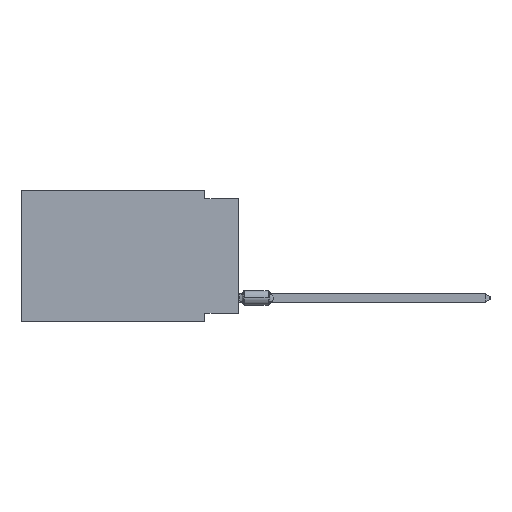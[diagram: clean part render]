
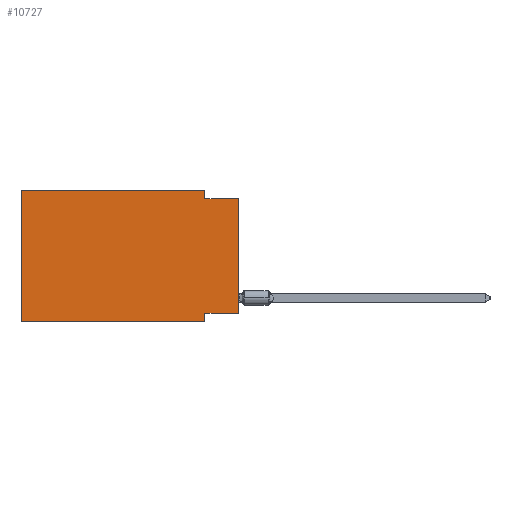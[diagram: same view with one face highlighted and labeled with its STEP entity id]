
A CAD part, left-side view. The second image highlights one B-rep face of the part: STEP entity #10727.
In plain terms, the highlighted planar face has unit normal (-1, 0, 0).
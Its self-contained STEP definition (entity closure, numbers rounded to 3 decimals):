
#38 = DIRECTION ( 'NONE',  ( 0., -1., 0. ) ) ;
#2158 = CARTESIAN_POINT ( 'NONE',  ( 0., 16.383, -9.906 ) ) ;
#3674 = LINE ( 'NONE', #37929, #44099 ) ;
#4008 = VECTOR ( 'NONE', #38, 1000. ) ;
#4027 = LINE ( 'NONE', #27089, #20086 ) ;
#5139 = CARTESIAN_POINT ( 'NONE',  ( 0., 0., -9.271 ) ) ;
#8320 = DIRECTION ( 'NONE',  ( 0., 0., 1. ) ) ;
#8462 = ORIENTED_EDGE ( 'NONE', *, *, #36257, .F. ) ;
#8533 = CARTESIAN_POINT ( 'NONE',  ( 0., 0., 0. ) ) ;
#8630 = DIRECTION ( 'NONE',  ( 1., 0., 0. ) ) ;
#8861 = FACE_OUTER_BOUND ( 'NONE', #24587, .T. ) ;
#9217 = ORIENTED_EDGE ( 'NONE', *, *, #28638, .F. ) ;
#10031 = VERTEX_POINT ( 'NONE', #24431 ) ;
#10727 = ADVANCED_FACE ( 'NONE', ( #8861 ), #39320, .F. ) ;
#11769 = CARTESIAN_POINT ( 'NONE',  ( 0., 16.383, 0. ) ) ;
#12430 = DIRECTION ( 'NONE',  ( 0., 0., -1. ) ) ;
#13097 = VECTOR ( 'NONE', #19785, 1000. ) ;
#13254 = VECTOR ( 'NONE', #38815, 1000. ) ;
#13742 = VECTOR ( 'NONE', #42339, 1000. ) ;
#15193 = ORIENTED_EDGE ( 'NONE', *, *, #21172, .F. ) ;
#15468 = EDGE_CURVE ( 'NONE', #16598, #10031, #3674, .T. ) ;
#16526 = ORIENTED_EDGE ( 'NONE', *, *, #15468, .F. ) ;
#16598 = VERTEX_POINT ( 'NONE', #39671 ) ;
#17488 = ORIENTED_EDGE ( 'NONE', *, *, #25750, .F. ) ;
#18610 = LINE ( 'NONE', #8533, #39622 ) ;
#18647 = CARTESIAN_POINT ( 'NONE',  ( 0., 16.383, 0. ) ) ;
#19785 = DIRECTION ( 'NONE',  ( 0., 1., 0. ) ) ;
#19995 = VERTEX_POINT ( 'NONE', #28957 ) ;
#20086 = VECTOR ( 'NONE', #20595, 1000. ) ;
#20595 = DIRECTION ( 'NONE',  ( 0., 0., -1. ) ) ;
#21172 = EDGE_CURVE ( 'NONE', #19995, #27235, #35238, .T. ) ;
#21295 = CARTESIAN_POINT ( 'NONE',  ( 0., 2.54, -9.906 ) ) ;
#21722 = CARTESIAN_POINT ( 'NONE',  ( 0., 2.54, -9.906 ) ) ;
#22419 = CARTESIAN_POINT ( 'NONE',  ( 0., 2.54, -9.271 ) ) ;
#23182 = CARTESIAN_POINT ( 'NONE',  ( 0., 16.383, 0. ) ) ;
#24431 = CARTESIAN_POINT ( 'NONE',  ( 0., 0., -0.635 ) ) ;
#24587 = EDGE_LOOP ( 'NONE', ( #43468, #16526, #17488, #9217, #15193, #35005, #26236, #8462 ) ) ;
#25228 = VERTEX_POINT ( 'NONE', #22419 ) ;
#25750 = EDGE_CURVE ( 'NONE', #42196, #16598, #4027, .T. ) ;
#26236 = ORIENTED_EDGE ( 'NONE', *, *, #33657, .F. ) ;
#27089 = CARTESIAN_POINT ( 'NONE',  ( 0., 2.54, 0. ) ) ;
#27235 = VERTEX_POINT ( 'NONE', #23182 ) ;
#28638 = EDGE_CURVE ( 'NONE', #27235, #42196, #36599, .T. ) ;
#28947 = VERTEX_POINT ( 'NONE', #5139 ) ;
#28957 = CARTESIAN_POINT ( 'NONE',  ( 0., 16.383, -9.906 ) ) ;
#29424 = VERTEX_POINT ( 'NONE', #21295 ) ;
#30718 = CARTESIAN_POINT ( 'NONE',  ( 0., 16.383, 0. ) ) ;
#31431 = DIRECTION ( 'NONE',  ( 0., -1., 0. ) ) ;
#31821 = EDGE_CURVE ( 'NONE', #19995, #29424, #35541, .T. ) ;
#32015 = AXIS2_PLACEMENT_3D ( 'NONE', #11769, #8630, #12430 ) ;
#33657 = EDGE_CURVE ( 'NONE', #25228, #29424, #42570, .T. ) ;
#33667 = CARTESIAN_POINT ( 'NONE',  ( 0., 0., -9.271 ) ) ;
#35005 = ORIENTED_EDGE ( 'NONE', *, *, #31821, .T. ) ;
#35238 = LINE ( 'NONE', #18647, #13254 ) ;
#35541 = LINE ( 'NONE', #2158, #40813 ) ;
#36257 = EDGE_CURVE ( 'NONE', #28947, #25228, #40408, .T. ) ;
#36599 = LINE ( 'NONE', #30718, #4008 ) ;
#37929 = CARTESIAN_POINT ( 'NONE',  ( 0., 0., -0.635 ) ) ;
#38815 = DIRECTION ( 'NONE',  ( 0., 0., 1. ) ) ;
#39131 = DIRECTION ( 'NONE',  ( 0., -1., 0. ) ) ;
#39320 = PLANE ( 'NONE',  #32015 ) ;
#39622 = VECTOR ( 'NONE', #8320, 1000. ) ;
#39671 = CARTESIAN_POINT ( 'NONE',  ( 0., 2.54, -0.635 ) ) ;
#40408 = LINE ( 'NONE', #33667, #13097 ) ;
#40813 = VECTOR ( 'NONE', #39131, 1000. ) ;
#41943 = CARTESIAN_POINT ( 'NONE',  ( 0., 2.54, 0. ) ) ;
#42196 = VERTEX_POINT ( 'NONE', #41943 ) ;
#42339 = DIRECTION ( 'NONE',  ( 0., 0., -1. ) ) ;
#42570 = LINE ( 'NONE', #21722, #13742 ) ;
#43468 = ORIENTED_EDGE ( 'NONE', *, *, #43520, .T. ) ;
#43520 = EDGE_CURVE ( 'NONE', #28947, #10031, #18610, .T. ) ;
#44099 = VECTOR ( 'NONE', #31431, 1000. ) ;
